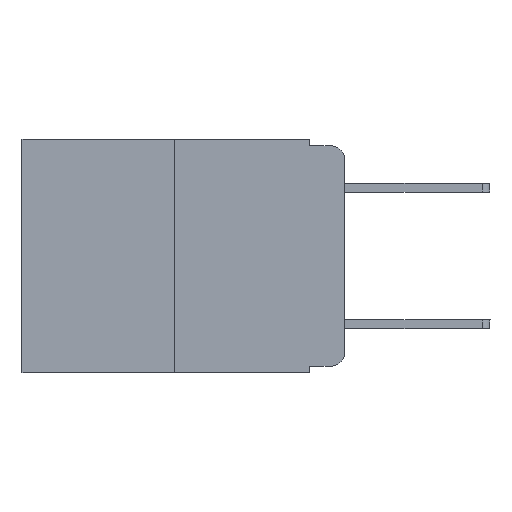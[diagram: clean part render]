
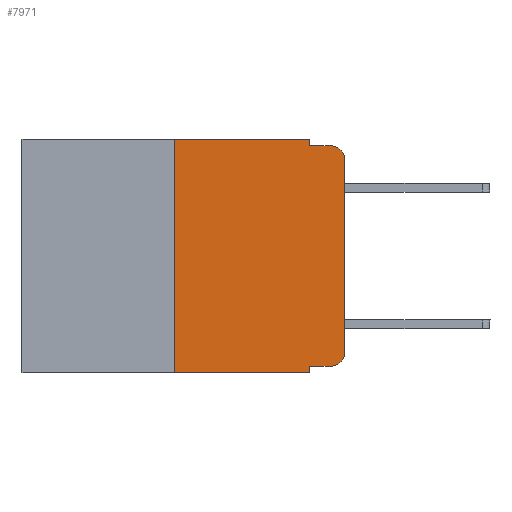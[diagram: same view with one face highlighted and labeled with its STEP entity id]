
A CAD part, left-side view. The second image highlights one B-rep face of the part: STEP entity #7971.
In plain terms, the highlighted planar face has unit normal (-1, 0, 0).
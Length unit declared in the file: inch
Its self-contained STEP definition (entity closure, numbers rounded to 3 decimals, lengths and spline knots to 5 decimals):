
#28 = DIRECTION ( 'NONE',  ( -1., 0., 0. ) ) ;
#607 = EDGE_CURVE ( 'NONE', #18634, #10999, #13019, .T. ) ;
#965 = CARTESIAN_POINT ( 'NONE',  ( 0., 0.473, -0.343 ) ) ;
#1014 = ORIENTED_EDGE ( 'NONE', *, *, #22624, .T. ) ;
#1154 = CIRCLE ( 'NONE', #19609, 0.02 ) ;
#1267 = EDGE_CURVE ( 'NONE', #22104, #16403, #18527, .T. ) ;
#1439 = EDGE_CURVE ( 'NONE', #15983, #10999, #1154, .T. ) ;
#1579 = AXIS2_PLACEMENT_3D ( 'NONE', #8118, #11598, #13461 ) ;
#1771 = DIRECTION ( 'NONE',  ( 0., -1., 0. ) ) ;
#1832 = DIRECTION ( 'NONE',  ( 0., 0., -1. ) ) ;
#1835 = LINE ( 'NONE', #11106, #20318 ) ;
#2454 = LINE ( 'NONE', #965, #11460 ) ;
#3681 = ORIENTED_EDGE ( 'NONE', *, *, #4273, .F. ) ;
#3764 = VERTEX_POINT ( 'NONE', #10855 ) ;
#3878 = EDGE_CURVE ( 'NONE', #19314, #6086, #22606, .T. ) ;
#4273 = EDGE_CURVE ( 'NONE', #9301, #19314, #1835, .T. ) ;
#5790 = ORIENTED_EDGE ( 'NONE', *, *, #23075, .T. ) ;
#6086 = VERTEX_POINT ( 'NONE', #11155 ) ;
#6260 = PLANE ( 'NONE',  #1579 ) ;
#7006 = EDGE_LOOP ( 'NONE', ( #18235, #7970, #12740, #11913, #21403, #3681, #5790, #18464, #1014, #22678 ) ) ;
#7475 = CARTESIAN_POINT ( 'NONE',  ( 0., 0.02, -0.313 ) ) ;
#7828 = CARTESIAN_POINT ( 'NONE',  ( 0., 0.25, 0. ) ) ;
#7970 = ORIENTED_EDGE ( 'NONE', *, *, #1439, .T. ) ;
#7971 = ADVANCED_FACE ( 'NONE', ( #15974 ), #6260, .F. ) ;
#8031 = DIRECTION ( 'NONE',  ( 0., -1., 0. ) ) ;
#8118 = CARTESIAN_POINT ( 'NONE',  ( 0., 0.473, 0. ) ) ;
#8353 = DIRECTION ( 'NONE',  ( 0., 0., -1. ) ) ;
#8707 = DIRECTION ( 'NONE',  ( 0., 0., -1. ) ) ;
#9301 = VERTEX_POINT ( 'NONE', #18950 ) ;
#9829 = CARTESIAN_POINT ( 'NONE',  ( 0., 0.02, -0.01 ) ) ;
#10219 = LINE ( 'NONE', #15812, #11332 ) ;
#10855 = CARTESIAN_POINT ( 'NONE',  ( 0., 0.051, -0.343 ) ) ;
#10898 = CARTESIAN_POINT ( 'NONE',  ( 0., 0.02, -0.333 ) ) ;
#10999 = VERTEX_POINT ( 'NONE', #9829 ) ;
#11106 = CARTESIAN_POINT ( 'NONE',  ( 0., 0.25, 0. ) ) ;
#11155 = CARTESIAN_POINT ( 'NONE',  ( 0., 0.051, 0. ) ) ;
#11332 = VECTOR ( 'NONE', #8707, 39.37008 ) ;
#11460 = VECTOR ( 'NONE', #18908, 39.37008 ) ;
#11598 = DIRECTION ( 'NONE',  ( 1., 0., 0. ) ) ;
#11913 = ORIENTED_EDGE ( 'NONE', *, *, #18059, .F. ) ;
#12558 = CARTESIAN_POINT ( 'NONE',  ( 0., 0.051, -0.333 ) ) ;
#12720 = VECTOR ( 'NONE', #20032, 39.37008 ) ;
#12740 = ORIENTED_EDGE ( 'NONE', *, *, #607, .F. ) ;
#13019 = LINE ( 'NONE', #17309, #14967 ) ;
#13188 = AXIS2_PLACEMENT_3D ( 'NONE', #7475, #28, #1832 ) ;
#13461 = DIRECTION ( 'NONE',  ( 0., 0., -1. ) ) ;
#13951 = CARTESIAN_POINT ( 'NONE',  ( 0., 0., -0.03 ) ) ;
#14209 = CARTESIAN_POINT ( 'NONE',  ( 0., 0.02, -0.03 ) ) ;
#14967 = VECTOR ( 'NONE', #15365, 39.37008 ) ;
#15365 = DIRECTION ( 'NONE',  ( 0., -1., 0. ) ) ;
#15767 = LINE ( 'NONE', #21980, #12720 ) ;
#15812 = CARTESIAN_POINT ( 'NONE',  ( 0., 0.051, 0. ) ) ;
#15974 = FACE_OUTER_BOUND ( 'NONE', #7006, .T. ) ;
#15983 = VERTEX_POINT ( 'NONE', #13951 ) ;
#16060 = DIRECTION ( 'NONE',  ( -1., 0., 0. ) ) ;
#16343 = CARTESIAN_POINT ( 'NONE',  ( 0., 0.051, -0.333 ) ) ;
#16403 = VERTEX_POINT ( 'NONE', #22024 ) ;
#17309 = CARTESIAN_POINT ( 'NONE',  ( 0., 0.051, -0.01 ) ) ;
#17739 = VERTEX_POINT ( 'NONE', #16343 ) ;
#18059 = EDGE_CURVE ( 'NONE', #6086, #18634, #23144, .T. ) ;
#18235 = ORIENTED_EDGE ( 'NONE', *, *, #20379, .T. ) ;
#18414 = CARTESIAN_POINT ( 'NONE',  ( 0., 0.051, -0.01 ) ) ;
#18464 = ORIENTED_EDGE ( 'NONE', *, *, #19596, .F. ) ;
#18471 = VECTOR ( 'NONE', #1771, 39.37008 ) ;
#18527 = CIRCLE ( 'NONE', #13188, 0.02 ) ;
#18634 = VERTEX_POINT ( 'NONE', #18414 ) ;
#18908 = DIRECTION ( 'NONE',  ( 0., -1., 0. ) ) ;
#18950 = CARTESIAN_POINT ( 'NONE',  ( 0., 0.25, -0.343 ) ) ;
#19314 = VERTEX_POINT ( 'NONE', #7828 ) ;
#19525 = VECTOR ( 'NONE', #8031, 39.37008 ) ;
#19596 = EDGE_CURVE ( 'NONE', #17739, #3764, #10219, .T. ) ;
#19609 = AXIS2_PLACEMENT_3D ( 'NONE', #14209, #16060, #23022 ) ;
#20032 = DIRECTION ( 'NONE',  ( 0., 0., 1. ) ) ;
#20318 = VECTOR ( 'NONE', #21708, 39.37008 ) ;
#20379 = EDGE_CURVE ( 'NONE', #16403, #15983, #15767, .T. ) ;
#20547 = CARTESIAN_POINT ( 'NONE',  ( 0., 0.051, 0. ) ) ;
#21185 = VECTOR ( 'NONE', #8353, 39.37008 ) ;
#21403 = ORIENTED_EDGE ( 'NONE', *, *, #3878, .F. ) ;
#21541 = LINE ( 'NONE', #12558, #18471 ) ;
#21708 = DIRECTION ( 'NONE',  ( 0., 0., 1. ) ) ;
#21980 = CARTESIAN_POINT ( 'NONE',  ( 0., 0., 0. ) ) ;
#22024 = CARTESIAN_POINT ( 'NONE',  ( 0., 0., -0.313 ) ) ;
#22104 = VERTEX_POINT ( 'NONE', #10898 ) ;
#22338 = CARTESIAN_POINT ( 'NONE',  ( 0., 0.473, 0. ) ) ;
#22606 = LINE ( 'NONE', #22338, #19525 ) ;
#22624 = EDGE_CURVE ( 'NONE', #17739, #22104, #21541, .T. ) ;
#22678 = ORIENTED_EDGE ( 'NONE', *, *, #1267, .T. ) ;
#23022 = DIRECTION ( 'NONE',  ( 0., 0., -1. ) ) ;
#23075 = EDGE_CURVE ( 'NONE', #9301, #3764, #2454, .T. ) ;
#23144 = LINE ( 'NONE', #20547, #21185 ) ;
